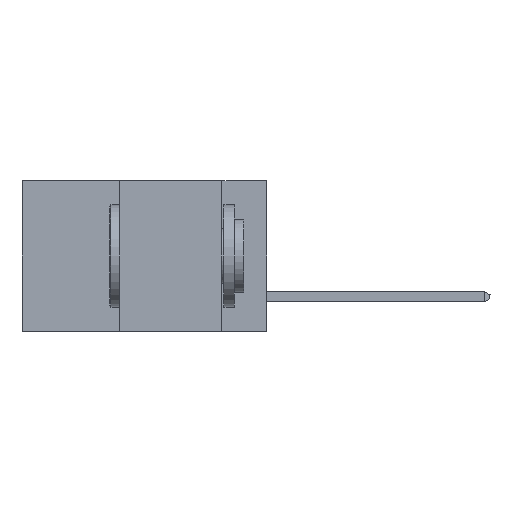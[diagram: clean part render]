
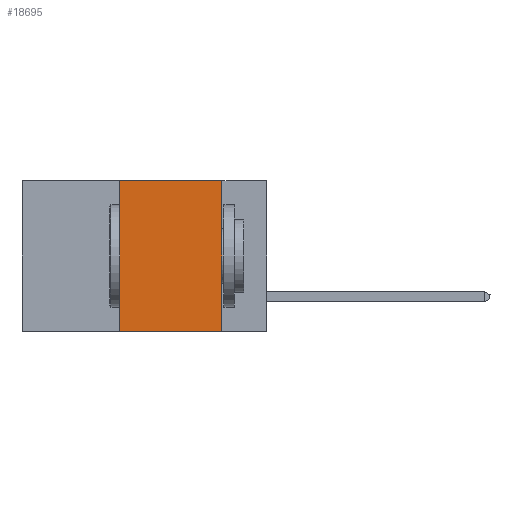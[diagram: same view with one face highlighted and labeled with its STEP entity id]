
A CAD part, left-side view. The second image highlights one B-rep face of the part: STEP entity #18695.
In plain terms, the highlighted planar face has unit normal (-1, 0, 0).
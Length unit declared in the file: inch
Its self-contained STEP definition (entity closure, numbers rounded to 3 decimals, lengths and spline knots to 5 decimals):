
#840 = VERTEX_POINT ( 'NONE', #3635 ) ;
#3183 = LINE ( 'NONE', #32404, #32741 ) ;
#3188 = VECTOR ( 'NONE', #41394, 39.37008 ) ;
#3635 = CARTESIAN_POINT ( 'NONE',  ( 0., 0.11, -0.37 ) ) ;
#7001 = CARTESIAN_POINT ( 'NONE',  ( 0., 0.6, 0. ) ) ;
#7944 = LINE ( 'NONE', #7001, #44069 ) ;
#10870 = EDGE_CURVE ( 'NONE', #17179, #22849, #7944, .T. ) ;
#10882 = CARTESIAN_POINT ( 'NONE',  ( 0., 0.36, 0. ) ) ;
#11861 = AXIS2_PLACEMENT_3D ( 'NONE', #22220, #29124, #39724 ) ;
#12067 = CARTESIAN_POINT ( 'NONE',  ( 0., 0.6, -0.37 ) ) ;
#12401 = CARTESIAN_POINT ( 'NONE',  ( 0., 0.36, -0.37 ) ) ;
#13115 = VECTOR ( 'NONE', #15856, 39.37008 ) ;
#15398 = ORIENTED_EDGE ( 'NONE', *, *, #10870, .F. ) ;
#15856 = DIRECTION ( 'NONE',  ( 0., -1., 0. ) ) ;
#17123 = ORIENTED_EDGE ( 'NONE', *, *, #40232, .F. ) ;
#17179 = VERTEX_POINT ( 'NONE', #10882 ) ;
#18695 = ADVANCED_FACE ( 'NONE', ( #28821 ), #28817, .F. ) ;
#21242 = EDGE_CURVE ( 'NONE', #42917, #840, #41642, .T. ) ;
#22220 = CARTESIAN_POINT ( 'NONE',  ( 0., 0.6, 0. ) ) ;
#22849 = VERTEX_POINT ( 'NONE', #43138 ) ;
#25172 = ORIENTED_EDGE ( 'NONE', *, *, #33107, .F. ) ;
#27225 = CARTESIAN_POINT ( 'NONE',  ( 0., 0.36, 0. ) ) ;
#27432 = EDGE_LOOP ( 'NONE', ( #17123, #15398, #25172, #29349 ) ) ;
#27757 = LINE ( 'NONE', #27225, #3188 ) ;
#28817 = PLANE ( 'NONE',  #11861 ) ;
#28821 = FACE_OUTER_BOUND ( 'NONE', #27432, .T. ) ;
#29124 = DIRECTION ( 'NONE',  ( 1., 0., 0. ) ) ;
#29349 = ORIENTED_EDGE ( 'NONE', *, *, #21242, .T. ) ;
#32404 = CARTESIAN_POINT ( 'NONE',  ( 0., 0.11, 0. ) ) ;
#32741 = VECTOR ( 'NONE', #39129, 39.37008 ) ;
#33107 = EDGE_CURVE ( 'NONE', #42917, #17179, #27757, .T. ) ;
#34727 = DIRECTION ( 'NONE',  ( 0., -1., 0. ) ) ;
#39129 = DIRECTION ( 'NONE',  ( 0., 0., -1. ) ) ;
#39724 = DIRECTION ( 'NONE',  ( 0., 0., -1. ) ) ;
#40232 = EDGE_CURVE ( 'NONE', #22849, #840, #3183, .T. ) ;
#41394 = DIRECTION ( 'NONE',  ( 0., 0., 1. ) ) ;
#41642 = LINE ( 'NONE', #12067, #13115 ) ;
#42917 = VERTEX_POINT ( 'NONE', #12401 ) ;
#43138 = CARTESIAN_POINT ( 'NONE',  ( 0., 0.11, 0. ) ) ;
#44069 = VECTOR ( 'NONE', #34727, 39.37008 ) ;
